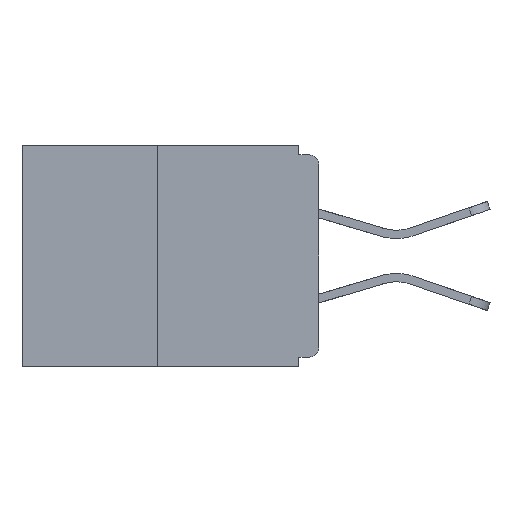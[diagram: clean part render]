
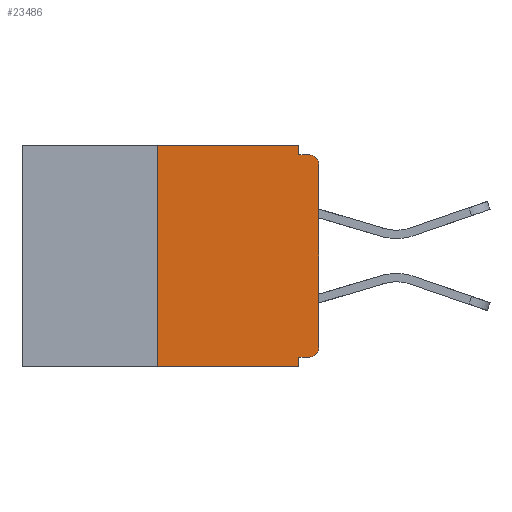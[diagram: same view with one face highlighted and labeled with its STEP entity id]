
A CAD part, left-side view. The second image highlights one B-rep face of the part: STEP entity #23486.
In plain terms, the highlighted planar face has unit normal (-1, 0, 0).
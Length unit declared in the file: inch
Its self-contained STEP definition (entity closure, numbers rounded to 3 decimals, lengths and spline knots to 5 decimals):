
#134 = PLANE ( 'NONE',  #8609 ) ;
#1025 = EDGE_CURVE ( 'NONE', #11698, #18028, #23972, .T. ) ;
#1130 = AXIS2_PLACEMENT_3D ( 'NONE', #10133, #7875, #8075 ) ;
#1378 = CARTESIAN_POINT ( 'NONE',  ( 0., 0.015, -0.328 ) ) ;
#1394 = CARTESIAN_POINT ( 'NONE',  ( 0., 0.031, -0.015 ) ) ;
#1515 = VECTOR ( 'NONE', #12799, 39.37008 ) ;
#1636 = DIRECTION ( 'NONE',  ( 0., 0., -1. ) ) ;
#1837 = LINE ( 'NONE', #9496, #18944 ) ;
#2057 = ORIENTED_EDGE ( 'NONE', *, *, #1025, .F. ) ;
#2125 = VECTOR ( 'NONE', #11388, 39.37008 ) ;
#2440 = EDGE_CURVE ( 'NONE', #10503, #6518, #4249, .T. ) ;
#3054 = LINE ( 'NONE', #19327, #26202 ) ;
#4249 = CIRCLE ( 'NONE', #1130, 0.015 ) ;
#4268 = VERTEX_POINT ( 'NONE', #1394 ) ;
#4541 = CARTESIAN_POINT ( 'NONE',  ( 0., 0.031, -0.343 ) ) ;
#4720 = CARTESIAN_POINT ( 'NONE',  ( 0., 0.031, -0.343 ) ) ;
#5048 = ORIENTED_EDGE ( 'NONE', *, *, #19498, .F. ) ;
#5119 = LINE ( 'NONE', #14826, #14877 ) ;
#5714 = VECTOR ( 'NONE', #17476, 39.37008 ) ;
#5877 = DIRECTION ( 'NONE',  ( 0., 0., 1. ) ) ;
#6053 = ORIENTED_EDGE ( 'NONE', *, *, #8275, .T. ) ;
#6310 = DIRECTION ( 'NONE',  ( 0., -1., 0. ) ) ;
#6437 = EDGE_LOOP ( 'NONE', ( #11765, #2057, #14196, #18928, #5048, #16002, #7265, #6053, #6728, #9975 ) ) ;
#6504 = CARTESIAN_POINT ( 'NONE',  ( 0., 0.015, -0.03 ) ) ;
#6518 = VERTEX_POINT ( 'NONE', #12729 ) ;
#6613 = FACE_OUTER_BOUND ( 'NONE', #6437, .T. ) ;
#6728 = ORIENTED_EDGE ( 'NONE', *, *, #21062, .F. ) ;
#6917 = VERTEX_POINT ( 'NONE', #28030 ) ;
#7027 = DIRECTION ( 'NONE',  ( 0., 0., -1. ) ) ;
#7265 = ORIENTED_EDGE ( 'NONE', *, *, #8910, .T. ) ;
#7835 = CARTESIAN_POINT ( 'NONE',  ( 0., 0.031, -0.328 ) ) ;
#7875 = DIRECTION ( 'NONE',  ( -1., 0., 0. ) ) ;
#8075 = DIRECTION ( 'NONE',  ( 0., 0., -1. ) ) ;
#8275 = EDGE_CURVE ( 'NONE', #6917, #13771, #20734, .T. ) ;
#8301 = CARTESIAN_POINT ( 'NONE',  ( 0., 0.015, -0.015 ) ) ;
#8465 = VERTEX_POINT ( 'NONE', #7835 ) ;
#8609 = AXIS2_PLACEMENT_3D ( 'NONE', #8897, #9099, #7027 ) ;
#8835 = DIRECTION ( 'NONE',  ( -1., 0., 0. ) ) ;
#8897 = CARTESIAN_POINT ( 'NONE',  ( 0., 0.46, 0. ) ) ;
#8910 = EDGE_CURVE ( 'NONE', #6518, #6917, #1837, .T. ) ;
#9099 = DIRECTION ( 'NONE',  ( 1., 0., 0. ) ) ;
#9496 = CARTESIAN_POINT ( 'NONE',  ( 0., 0., 0. ) ) ;
#9686 = DIRECTION ( 'NONE',  ( 0., 0., -1. ) ) ;
#9975 = ORIENTED_EDGE ( 'NONE', *, *, #17065, .F. ) ;
#10133 = CARTESIAN_POINT ( 'NONE',  ( 0., 0.015, -0.313 ) ) ;
#10392 = LINE ( 'NONE', #4541, #11791 ) ;
#10503 = VERTEX_POINT ( 'NONE', #1378 ) ;
#11338 = CARTESIAN_POINT ( 'NONE',  ( 0., 0.25, 0. ) ) ;
#11388 = DIRECTION ( 'NONE',  ( 0., -1., 0. ) ) ;
#11698 = VERTEX_POINT ( 'NONE', #26480 ) ;
#11765 = ORIENTED_EDGE ( 'NONE', *, *, #22155, .F. ) ;
#11791 = VECTOR ( 'NONE', #9686, 39.37008 ) ;
#12729 = CARTESIAN_POINT ( 'NONE',  ( 0., 0., -0.313 ) ) ;
#12799 = DIRECTION ( 'NONE',  ( 0., 1., 0. ) ) ;
#13701 = DIRECTION ( 'NONE',  ( 0., 0., 1. ) ) ;
#13771 = VERTEX_POINT ( 'NONE', #8301 ) ;
#14196 = ORIENTED_EDGE ( 'NONE', *, *, #15454, .T. ) ;
#14442 = VECTOR ( 'NONE', #5877, 39.37008 ) ;
#14648 = LINE ( 'NONE', #24422, #2125 ) ;
#14826 = CARTESIAN_POINT ( 'NONE',  ( 0., 0.031, 0. ) ) ;
#14877 = VECTOR ( 'NONE', #20448, 39.37008 ) ;
#15454 = EDGE_CURVE ( 'NONE', #11698, #23037, #15826, .T. ) ;
#15826 = LINE ( 'NONE', #24162, #5714 ) ;
#16002 = ORIENTED_EDGE ( 'NONE', *, *, #2440, .T. ) ;
#17065 = EDGE_CURVE ( 'NONE', #20194, #4268, #5119, .T. ) ;
#17228 = LINE ( 'NONE', #28323, #1515 ) ;
#17298 = CARTESIAN_POINT ( 'NONE',  ( 0., 0.031, 0. ) ) ;
#17476 = DIRECTION ( 'NONE',  ( 0., -1., 0. ) ) ;
#18028 = VERTEX_POINT ( 'NONE', #11338 ) ;
#18928 = ORIENTED_EDGE ( 'NONE', *, *, #27943, .F. ) ;
#18944 = VECTOR ( 'NONE', #13701, 39.37008 ) ;
#19327 = CARTESIAN_POINT ( 'NONE',  ( 0., 0.46, 0. ) ) ;
#19498 = EDGE_CURVE ( 'NONE', #10503, #8465, #17228, .T. ) ;
#20194 = VERTEX_POINT ( 'NONE', #17298 ) ;
#20448 = DIRECTION ( 'NONE',  ( 0., 0., -1. ) ) ;
#20734 = CIRCLE ( 'NONE', #22984, 0.015 ) ;
#21062 = EDGE_CURVE ( 'NONE', #4268, #13771, #14648, .T. ) ;
#21343 = CARTESIAN_POINT ( 'NONE',  ( 0., 0.25, 0. ) ) ;
#22155 = EDGE_CURVE ( 'NONE', #18028, #20194, #3054, .T. ) ;
#22984 = AXIS2_PLACEMENT_3D ( 'NONE', #6504, #8835, #1636 ) ;
#23037 = VERTEX_POINT ( 'NONE', #4720 ) ;
#23486 = ADVANCED_FACE ( 'NONE', ( #6613 ), #134, .F. ) ;
#23972 = LINE ( 'NONE', #21343, #14442 ) ;
#24162 = CARTESIAN_POINT ( 'NONE',  ( 0., 0.46, -0.343 ) ) ;
#24422 = CARTESIAN_POINT ( 'NONE',  ( 0., 0., -0.015 ) ) ;
#26202 = VECTOR ( 'NONE', #6310, 39.37008 ) ;
#26480 = CARTESIAN_POINT ( 'NONE',  ( 0., 0.25, -0.343 ) ) ;
#27943 = EDGE_CURVE ( 'NONE', #8465, #23037, #10392, .T. ) ;
#28030 = CARTESIAN_POINT ( 'NONE',  ( 0., 0., -0.03 ) ) ;
#28323 = CARTESIAN_POINT ( 'NONE',  ( 0., 0., -0.328 ) ) ;
